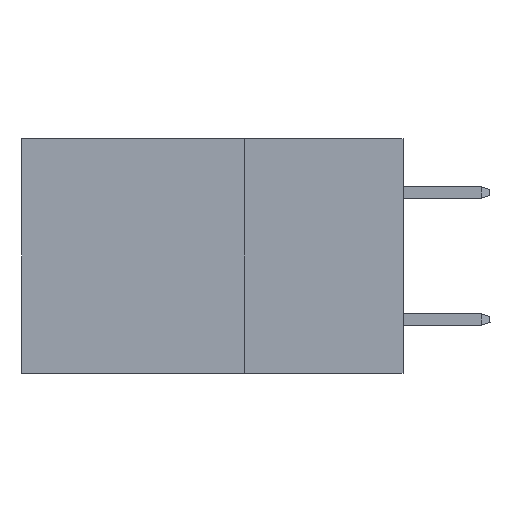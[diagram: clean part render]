
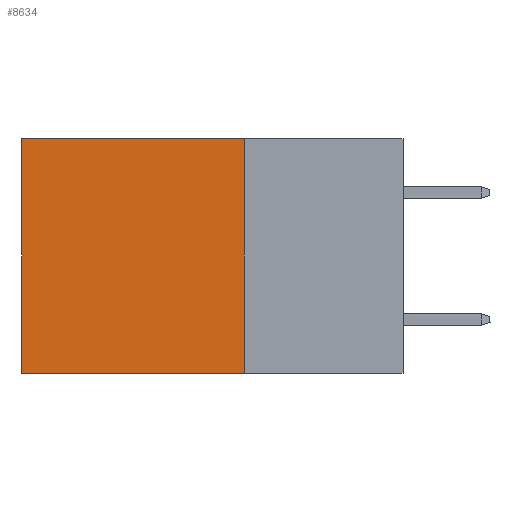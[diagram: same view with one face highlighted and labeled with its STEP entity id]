
A CAD part, left-side view. The second image highlights one B-rep face of the part: STEP entity #8634.
In plain terms, the highlighted planar face has unit normal (-1, 0, 0).
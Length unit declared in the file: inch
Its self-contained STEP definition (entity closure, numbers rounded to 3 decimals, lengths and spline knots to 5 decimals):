
#141 = CARTESIAN_POINT ( 'NONE',  ( 0.2875, 0.25, -0.37 ) ) ;
#271 = PLANE ( 'NONE',  #5415 ) ;
#464 = LINE ( 'NONE', #4433, #12266 ) ;
#1157 = DIRECTION ( 'NONE',  ( 0., 1., 0. ) ) ;
#1225 = EDGE_CURVE ( 'NONE', #3480, #12468, #5929, .T. ) ;
#1361 = CARTESIAN_POINT ( 'NONE',  ( 0.2875, 0.25, 0. ) ) ;
#1439 = VERTEX_POINT ( 'NONE', #11348 ) ;
#2319 = VECTOR ( 'NONE', #1157, 39.37008 ) ;
#2509 = DIRECTION ( 'NONE',  ( 0., 0., -1. ) ) ;
#3480 = VERTEX_POINT ( 'NONE', #9675 ) ;
#3486 = EDGE_CURVE ( 'NONE', #9798, #1439, #464, .T. ) ;
#3924 = ORIENTED_EDGE ( 'NONE', *, *, #6368, .T. ) ;
#4322 = DIRECTION ( 'NONE',  ( 0., 1., 0. ) ) ;
#4433 = CARTESIAN_POINT ( 'NONE',  ( 0.2875, 0.6, 0. ) ) ;
#4654 = ORIENTED_EDGE ( 'NONE', *, *, #3486, .T. ) ;
#4961 = DIRECTION ( 'NONE',  ( 0., 0., -1. ) ) ;
#5359 = LINE ( 'NONE', #141, #11574 ) ;
#5415 = AXIS2_PLACEMENT_3D ( 'NONE', #1361, #10986, #2509 ) ;
#5797 = CARTESIAN_POINT ( 'NONE',  ( 0.2875, 0.25, 0. ) ) ;
#5929 = LINE ( 'NONE', #5797, #7615 ) ;
#6305 = ORIENTED_EDGE ( 'NONE', *, *, #9185, .F. ) ;
#6368 = EDGE_CURVE ( 'NONE', #3480, #9798, #7395, .T. ) ;
#7395 = LINE ( 'NONE', #10560, #2319 ) ;
#7615 = VECTOR ( 'NONE', #4961, 39.37008 ) ;
#7620 = FACE_OUTER_BOUND ( 'NONE', #9604, .T. ) ;
#8581 = DIRECTION ( 'NONE',  ( 0., 0., -1. ) ) ;
#8634 = ADVANCED_FACE ( 'NONE', ( #7620 ), #271, .F. ) ;
#9185 = EDGE_CURVE ( 'NONE', #12468, #1439, #5359, .T. ) ;
#9604 = EDGE_LOOP ( 'NONE', ( #4654, #6305, #10428, #3924 ) ) ;
#9675 = CARTESIAN_POINT ( 'NONE',  ( 0.2875, 0.25, 0. ) ) ;
#9798 = VERTEX_POINT ( 'NONE', #11554 ) ;
#10428 = ORIENTED_EDGE ( 'NONE', *, *, #1225, .F. ) ;
#10560 = CARTESIAN_POINT ( 'NONE',  ( 0.2875, 0.25, 0. ) ) ;
#10986 = DIRECTION ( 'NONE',  ( 1., 0., 0. ) ) ;
#11273 = CARTESIAN_POINT ( 'NONE',  ( 0.2875, 0.25, -0.37 ) ) ;
#11348 = CARTESIAN_POINT ( 'NONE',  ( 0.2875, 0.6, -0.37 ) ) ;
#11554 = CARTESIAN_POINT ( 'NONE',  ( 0.2875, 0.6, 0. ) ) ;
#11574 = VECTOR ( 'NONE', #4322, 39.37008 ) ;
#12266 = VECTOR ( 'NONE', #8581, 39.37008 ) ;
#12468 = VERTEX_POINT ( 'NONE', #11273 ) ;
